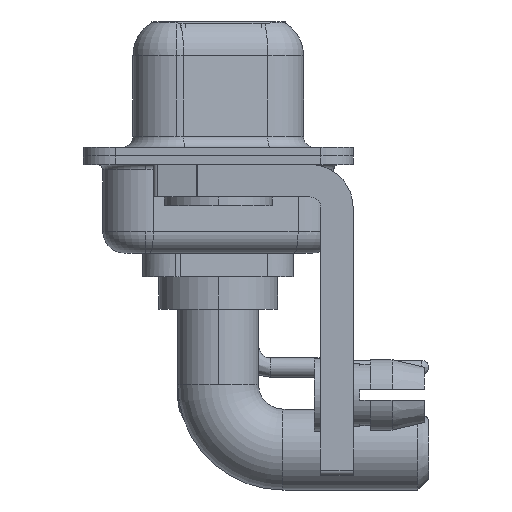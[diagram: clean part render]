
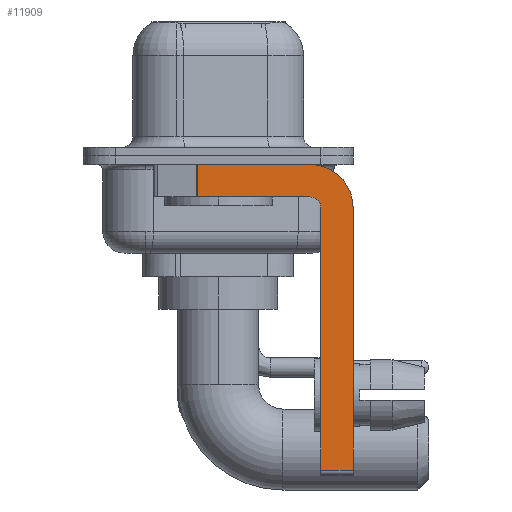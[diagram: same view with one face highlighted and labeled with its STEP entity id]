
A CAD part, left-side view. The second image highlights one B-rep face of the part: STEP entity #11909.
In plain terms, the highlighted planar face has unit normal (-1, 0, 0).
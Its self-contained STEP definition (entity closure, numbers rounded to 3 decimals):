
#763 = DIRECTION ( 'NONE',  ( 0., 0., 1. ) ) ;
#989 = CARTESIAN_POINT ( 'NONE',  ( -2.9, -4.25, -1.9 ) ) ;
#1030 = FACE_OUTER_BOUND ( 'NONE', #2624, .T. ) ;
#1216 = VERTEX_POINT ( 'NONE', #23614 ) ;
#1533 = ORIENTED_EDGE ( 'NONE', *, *, #24462, .T. ) ;
#1714 = LINE ( 'NONE', #7695, #11457 ) ;
#1799 = CIRCLE ( 'NONE', #18303, 2. ) ;
#1898 = DIRECTION ( 'NONE',  ( 0., 1., 0. ) ) ;
#2077 = LINE ( 'NONE', #24352, #7823 ) ;
#2624 = EDGE_LOOP ( 'NONE', ( #23817, #5225, #21257, #4458, #24323, #1533, #5861, #24692 ) ) ;
#3398 = AXIS2_PLACEMENT_3D ( 'NONE', #8261, #6146, #24683 ) ;
#3635 = CARTESIAN_POINT ( 'NONE',  ( -2.9, -4.25, -1.9 ) ) ;
#3695 = VERTEX_POINT ( 'NONE', #6444 ) ;
#4247 = DIRECTION ( 'NONE',  ( 0., 0., -1. ) ) ;
#4458 = ORIENTED_EDGE ( 'NONE', *, *, #12553, .F. ) ;
#4482 = EDGE_CURVE ( 'NONE', #17903, #16396, #18200, .T. ) ;
#5215 = CARTESIAN_POINT ( 'NONE',  ( -2.9, -6.25, -14.55 ) ) ;
#5225 = ORIENTED_EDGE ( 'NONE', *, *, #11638, .T. ) ;
#5287 = CARTESIAN_POINT ( 'NONE',  ( -2.9, -6.25, -2.4 ) ) ;
#5861 = ORIENTED_EDGE ( 'NONE', *, *, #19419, .F. ) ;
#6146 = DIRECTION ( 'NONE',  ( -1., 0., 0. ) ) ;
#6444 = CARTESIAN_POINT ( 'NONE',  ( -2.9, -4.75, -2.4 ) ) ;
#6510 = CARTESIAN_POINT ( 'NONE',  ( -2.9, -4.75, -14.55 ) ) ;
#7608 = VECTOR ( 'NONE', #4247, 1000. ) ;
#7695 = CARTESIAN_POINT ( 'NONE',  ( -2.9, -4.25, -14.55 ) ) ;
#7823 = VECTOR ( 'NONE', #10829, 1000. ) ;
#7977 = VERTEX_POINT ( 'NONE', #5287 ) ;
#8053 = CIRCLE ( 'NONE', #3398, 0.5 ) ;
#8261 = CARTESIAN_POINT ( 'NONE',  ( -2.9, -4.25, -2.4 ) ) ;
#8847 = CARTESIAN_POINT ( 'NONE',  ( -2.9, 3., -0.4 ) ) ;
#9096 = EDGE_CURVE ( 'NONE', #22341, #3695, #9135, .T. ) ;
#9135 = LINE ( 'NONE', #18798, #16587 ) ;
#9142 = PLANE ( 'NONE',  #24945 ) ;
#9957 = CARTESIAN_POINT ( 'NONE',  ( -2.9, 0.978, -1.9 ) ) ;
#10296 = CARTESIAN_POINT ( 'NONE',  ( -2.9, 0.978, -1.9 ) ) ;
#10605 = DIRECTION ( 'NONE',  ( 1., 0., 0. ) ) ;
#10829 = DIRECTION ( 'NONE',  ( 0., 0., -1. ) ) ;
#10893 = DIRECTION ( 'NONE',  ( 0., 0., -1. ) ) ;
#11293 = EDGE_CURVE ( 'NONE', #23129, #7977, #1799, .T. ) ;
#11457 = VECTOR ( 'NONE', #21733, 1000. ) ;
#11638 = EDGE_CURVE ( 'NONE', #1216, #16396, #18148, .T. ) ;
#11909 = ADVANCED_FACE ( 'NONE', ( #1030 ), #9142, .F. ) ;
#12553 = EDGE_CURVE ( 'NONE', #3695, #17903, #8053, .T. ) ;
#14723 = EDGE_CURVE ( 'NONE', #1216, #23129, #16531, .T. ) ;
#16396 = VERTEX_POINT ( 'NONE', #10296 ) ;
#16531 = LINE ( 'NONE', #8847, #25868 ) ;
#16587 = VECTOR ( 'NONE', #763, 1000. ) ;
#17028 = VERTEX_POINT ( 'NONE', #5215 ) ;
#17210 = CARTESIAN_POINT ( 'NONE',  ( -2.9, -4.25, -2.4 ) ) ;
#17903 = VERTEX_POINT ( 'NONE', #989 ) ;
#18148 = LINE ( 'NONE', #9957, #7608 ) ;
#18200 = LINE ( 'NONE', #3635, #24916 ) ;
#18303 = AXIS2_PLACEMENT_3D ( 'NONE', #25201, #21086, #10893 ) ;
#18798 = CARTESIAN_POINT ( 'NONE',  ( -2.9, -4.75, -14.8 ) ) ;
#18805 = DIRECTION ( 'NONE',  ( 0., 0., -1. ) ) ;
#19419 = EDGE_CURVE ( 'NONE', #7977, #17028, #2077, .T. ) ;
#21086 = DIRECTION ( 'NONE',  ( 1., 0., 0. ) ) ;
#21257 = ORIENTED_EDGE ( 'NONE', *, *, #4482, .F. ) ;
#21733 = DIRECTION ( 'NONE',  ( 0., -1., 0. ) ) ;
#22341 = VERTEX_POINT ( 'NONE', #6510 ) ;
#23090 = CARTESIAN_POINT ( 'NONE',  ( -2.9, -4.25, -0.4 ) ) ;
#23129 = VERTEX_POINT ( 'NONE', #23090 ) ;
#23614 = CARTESIAN_POINT ( 'NONE',  ( -2.9, 0.978, -0.4 ) ) ;
#23817 = ORIENTED_EDGE ( 'NONE', *, *, #14723, .F. ) ;
#24323 = ORIENTED_EDGE ( 'NONE', *, *, #9096, .F. ) ;
#24352 = CARTESIAN_POINT ( 'NONE',  ( -2.9, -6.25, -2.4 ) ) ;
#24462 = EDGE_CURVE ( 'NONE', #22341, #17028, #1714, .T. ) ;
#24683 = DIRECTION ( 'NONE',  ( 0., 0., 1. ) ) ;
#24692 = ORIENTED_EDGE ( 'NONE', *, *, #11293, .F. ) ;
#24916 = VECTOR ( 'NONE', #1898, 1000. ) ;
#24945 = AXIS2_PLACEMENT_3D ( 'NONE', #17210, #10605, #18805 ) ;
#25011 = DIRECTION ( 'NONE',  ( 0., -1., 0. ) ) ;
#25201 = CARTESIAN_POINT ( 'NONE',  ( -2.9, -4.25, -2.4 ) ) ;
#25868 = VECTOR ( 'NONE', #25011, 1000. ) ;
